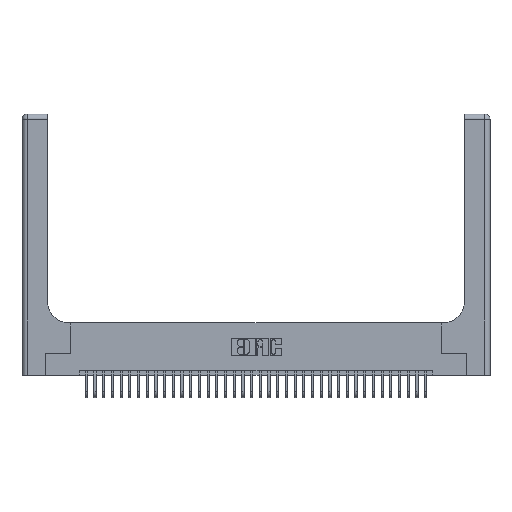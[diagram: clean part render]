
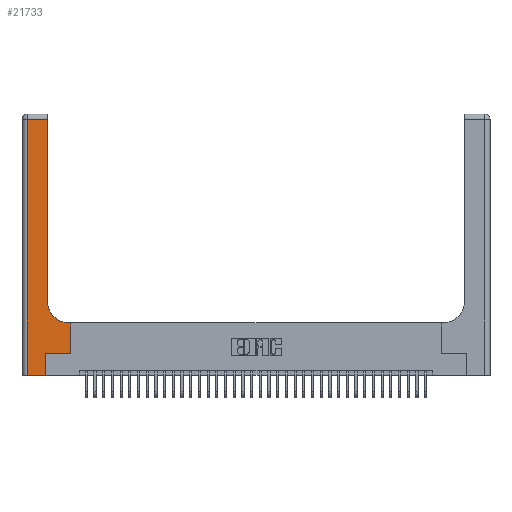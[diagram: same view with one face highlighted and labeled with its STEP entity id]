
A CAD part, top view. The second image highlights one B-rep face of the part: STEP entity #21733.
In plain terms, the highlighted planar face has unit normal (0, 0, 1).
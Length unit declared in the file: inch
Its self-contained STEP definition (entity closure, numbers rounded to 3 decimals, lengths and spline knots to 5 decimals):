
#333 = CARTESIAN_POINT ( 'NONE',  ( 0., 3., 0.37 ) ) ;
#889 = VERTEX_POINT ( 'NONE', #31517 ) ;
#1518 = CARTESIAN_POINT ( 'NONE',  ( 0.06, 2.94, 0.37 ) ) ;
#2050 = VERTEX_POINT ( 'NONE', #27858 ) ;
#2883 = EDGE_CURVE ( 'NONE', #12702, #31050, #9837, .T. ) ;
#3074 = DIRECTION ( 'NONE',  ( -1., 0., 0. ) ) ;
#3263 = VECTOR ( 'NONE', #3967, 39.37008 ) ;
#3561 = VERTEX_POINT ( 'NONE', #31207 ) ;
#3636 = CARTESIAN_POINT ( 'NONE',  ( 0.2915, 0.6, 0.37 ) ) ;
#3967 = DIRECTION ( 'NONE',  ( 0., -1., 0. ) ) ;
#4901 = DIRECTION ( 'NONE',  ( -1., 0., 0. ) ) ;
#5154 = LINE ( 'NONE', #17731, #19890 ) ;
#6546 = CARTESIAN_POINT ( 'NONE',  ( 0.2915, 2.94, 0.37 ) ) ;
#6815 = EDGE_CURVE ( 'NONE', #12469, #2050, #13869, .T. ) ;
#6817 = ORIENTED_EDGE ( 'NONE', *, *, #29501, .T. ) ;
#7001 = LINE ( 'NONE', #8839, #34529 ) ;
#7077 = EDGE_CURVE ( 'NONE', #31050, #9945, #26829, .T. ) ;
#7910 = CARTESIAN_POINT ( 'NONE',  ( 0.2915, 0.85, 0.37 ) ) ;
#8839 = CARTESIAN_POINT ( 'NONE',  ( 0.269, 0., 0.37 ) ) ;
#8867 = ORIENTED_EDGE ( 'NONE', *, *, #7077, .T. ) ;
#9482 = CARTESIAN_POINT ( 'NONE',  ( 0.2915, 3., 0.37 ) ) ;
#9837 = CIRCLE ( 'NONE', #23114, 0.25 ) ;
#9945 = VERTEX_POINT ( 'NONE', #6546 ) ;
#10637 = LINE ( 'NONE', #15005, #3263 ) ;
#11682 = CARTESIAN_POINT ( 'NONE',  ( 0.5585, 0.25, 0.37 ) ) ;
#12149 = VECTOR ( 'NONE', #19510, 39.37008 ) ;
#12469 = VERTEX_POINT ( 'NONE', #23357 ) ;
#12702 = VERTEX_POINT ( 'NONE', #18747 ) ;
#12849 = FACE_OUTER_BOUND ( 'NONE', #20121, .T. ) ;
#13226 = EDGE_CURVE ( 'NONE', #24568, #3561, #20803, .T. ) ;
#13869 = LINE ( 'NONE', #33137, #12149 ) ;
#14944 = DIRECTION ( 'NONE',  ( 0., 0., -1. ) ) ;
#15005 = CARTESIAN_POINT ( 'NONE',  ( 0.06, 3., 0.37 ) ) ;
#15456 = ORIENTED_EDGE ( 'NONE', *, *, #34269, .T. ) ;
#15469 = AXIS2_PLACEMENT_3D ( 'NONE', #333, #19653, #3074 ) ;
#15932 = LINE ( 'NONE', #3636, #29678 ) ;
#16068 = VECTOR ( 'NONE', #4901, 39.37008 ) ;
#17731 = CARTESIAN_POINT ( 'NONE',  ( 0.269, 0.25, 0.37 ) ) ;
#18700 = CARTESIAN_POINT ( 'NONE',  ( 0., 2.94, 0.37 ) ) ;
#18747 = CARTESIAN_POINT ( 'NONE',  ( 0.5415, 0.6, 0.37 ) ) ;
#19510 = DIRECTION ( 'NONE',  ( 1., 0., 0. ) ) ;
#19653 = DIRECTION ( 'NONE',  ( 0., 0., -1. ) ) ;
#19821 = DIRECTION ( 'NONE',  ( 0., 1., 0. ) ) ;
#19882 = DIRECTION ( 'NONE',  ( 0., 1., 0. ) ) ;
#19890 = VECTOR ( 'NONE', #20501, 39.37008 ) ;
#20121 = EDGE_LOOP ( 'NONE', ( #8867, #28402, #25453, #23381, #22224, #15456, #24878, #6817, #24256 ) ) ;
#20501 = DIRECTION ( 'NONE',  ( 1., 0., 0. ) ) ;
#20803 = LINE ( 'NONE', #11682, #27244 ) ;
#21298 = CARTESIAN_POINT ( 'NONE',  ( 0.5585, 0.25, 0.37 ) ) ;
#21733 = ADVANCED_FACE ( 'NONE', ( #12849 ), #33274, .F. ) ;
#21930 = VERTEX_POINT ( 'NONE', #1518 ) ;
#22224 = ORIENTED_EDGE ( 'NONE', *, *, #27491, .T. ) ;
#23114 = AXIS2_PLACEMENT_3D ( 'NONE', #31366, #14944, #34123 ) ;
#23219 = EDGE_CURVE ( 'NONE', #21930, #12469, #10637, .T. ) ;
#23357 = CARTESIAN_POINT ( 'NONE',  ( 0.06, 0., 0.37 ) ) ;
#23360 = DIRECTION ( 'NONE',  ( 0., 1., 0. ) ) ;
#23381 = ORIENTED_EDGE ( 'NONE', *, *, #6815, .T. ) ;
#23417 = LINE ( 'NONE', #18700, #16068 ) ;
#24256 = ORIENTED_EDGE ( 'NONE', *, *, #2883, .T. ) ;
#24568 = VERTEX_POINT ( 'NONE', #21298 ) ;
#24878 = ORIENTED_EDGE ( 'NONE', *, *, #13226, .T. ) ;
#25453 = ORIENTED_EDGE ( 'NONE', *, *, #23219, .T. ) ;
#25749 = DIRECTION ( 'NONE',  ( -1., 0., 0. ) ) ;
#26829 = LINE ( 'NONE', #9482, #33203 ) ;
#27244 = VECTOR ( 'NONE', #19882, 39.37008 ) ;
#27491 = EDGE_CURVE ( 'NONE', #2050, #889, #7001, .T. ) ;
#27858 = CARTESIAN_POINT ( 'NONE',  ( 0.269, 0., 0.37 ) ) ;
#27875 = EDGE_CURVE ( 'NONE', #9945, #21930, #23417, .T. ) ;
#28402 = ORIENTED_EDGE ( 'NONE', *, *, #27875, .T. ) ;
#29501 = EDGE_CURVE ( 'NONE', #3561, #12702, #15932, .T. ) ;
#29678 = VECTOR ( 'NONE', #25749, 39.37008 ) ;
#31050 = VERTEX_POINT ( 'NONE', #7910 ) ;
#31207 = CARTESIAN_POINT ( 'NONE',  ( 0.5585, 0.6, 0.37 ) ) ;
#31366 = CARTESIAN_POINT ( 'NONE',  ( 0.5415, 0.85, 0.37 ) ) ;
#31517 = CARTESIAN_POINT ( 'NONE',  ( 0.269, 0.25, 0.37 ) ) ;
#33137 = CARTESIAN_POINT ( 'NONE',  ( 0., 0., 0.37 ) ) ;
#33203 = VECTOR ( 'NONE', #23360, 39.37008 ) ;
#33274 = PLANE ( 'NONE',  #15469 ) ;
#34123 = DIRECTION ( 'NONE',  ( 1., 0., 0. ) ) ;
#34269 = EDGE_CURVE ( 'NONE', #889, #24568, #5154, .T. ) ;
#34529 = VECTOR ( 'NONE', #19821, 39.37008 ) ;
